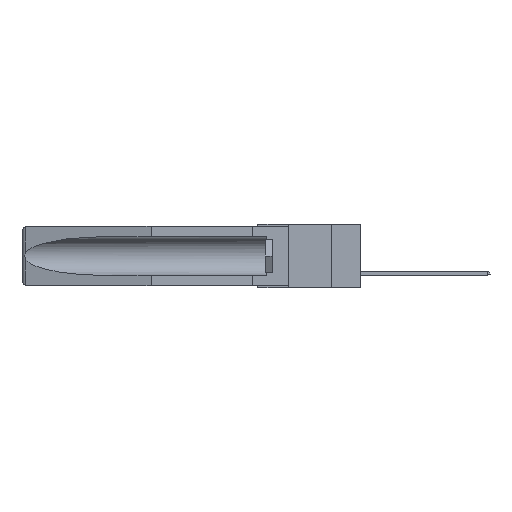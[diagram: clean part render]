
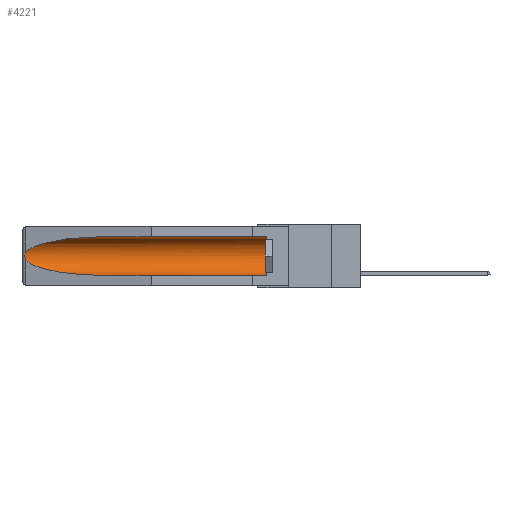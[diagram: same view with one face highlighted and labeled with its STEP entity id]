
A CAD part, left-side view. The second image highlights one B-rep face of the part: STEP entity #4221.
In plain terms, the highlighted cylindrical face has radius 2.857 mm (diameter 5.715 mm), a partial arc.
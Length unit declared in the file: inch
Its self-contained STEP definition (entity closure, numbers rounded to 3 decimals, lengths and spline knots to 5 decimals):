
#204 = VERTEX_POINT ( 'NONE', #32647 ) ;
#255 = EDGE_LOOP ( 'NONE', ( #9929, #26376, #19438, #7345, #10307, #28640 ) ) ;
#1029 = CARTESIAN_POINT ( 'NONE',  ( 0.26655, 1.53094, -0.18657 ) ) ;
#1532 =( BOUNDED_CURVE ( )  B_SPLINE_CURVE ( 3, ( #26139, #7770, #10874, #23546 ),
 .UNSPECIFIED., .F., .F. ) 
 B_SPLINE_CURVE_WITH_KNOTS ( ( 4, 4 ),
 ( 4.71239, 6.08839 ),
 .UNSPECIFIED. ) 
 CURVE ( )  GEOMETRIC_REPRESENTATION_ITEM ( )  RATIONAL_B_SPLINE_CURVE ( ( 1., 0.848, 0.848, 1. ) ) 
 REPRESENTATION_ITEM ( '' )  );
#1711 = DIRECTION ( 'NONE',  ( 0., 0., 1. ) ) ;
#2578 =( BOUNDED_CURVE ( )  B_SPLINE_CURVE ( 3, ( #14577, #17457, #25139, #32264 ),
 .UNSPECIFIED., .F., .F. ) 
 B_SPLINE_CURVE_WITH_KNOTS ( ( 4, 4 ),
 ( 0.1948, 1.5708 ),
 .UNSPECIFIED. ) 
 CURVE ( )  GEOMETRIC_REPRESENTATION_ITEM ( )  RATIONAL_B_SPLINE_CURVE ( ( 1., 0.848, 0.848, 1. ) ) 
 REPRESENTATION_ITEM ( '' )  );
#3154 = VERTEX_POINT ( 'NONE', #9610 ) ;
#3548 = DIRECTION ( 'NONE',  ( 0., -1., 0. ) ) ;
#4221 = ADVANCED_FACE ( 'NONE', ( #26932 ), #6598, .F. ) ;
#6135 = DIRECTION ( 'NONE',  ( 0., 1., 0. ) ) ;
#6598 = CYLINDRICAL_SURFACE ( 'NONE', #27250, 0.1125 ) ;
#7075 = CARTESIAN_POINT ( 'NONE',  ( 0.155, 1.07973, -0.284 ) ) ;
#7345 = ORIENTED_EDGE ( 'NONE', *, *, #27409, .F. ) ;
#7770 = CARTESIAN_POINT ( 'NONE',  ( 0.21114, 1.30732, -0.059 ) ) ;
#8404 = VERTEX_POINT ( 'NONE', #16386 ) ;
#8827 = CARTESIAN_POINT ( 'NONE',  ( 0.26597, 1.52961, -0.15275 ) ) ;
#9610 = CARTESIAN_POINT ( 'NONE',  ( 0.155, 0.126, -0.284 ) ) ;
#9929 = ORIENTED_EDGE ( 'NONE', *, *, #29488, .T. ) ;
#10307 = ORIENTED_EDGE ( 'NONE', *, *, #11218, .T. ) ;
#10533 = CARTESIAN_POINT ( 'NONE',  ( 0.26537, 1.52718, -0.19328 ) ) ;
#10874 = CARTESIAN_POINT ( 'NONE',  ( 0.25451, 1.48313, -0.09465 ) ) ;
#11218 = EDGE_CURVE ( 'NONE', #3154, #31500, #13970, .T. ) ;
#11290 = CARTESIAN_POINT ( 'NONE',  ( 0.2675, 1.53308, -0.16763 ) ) ;
#12491 = VERTEX_POINT ( 'NONE', #10533 ) ;
#13742 = CARTESIAN_POINT ( 'NONE',  ( 0.26537, 1.52718, -0.14972 ) ) ;
#13970 = CIRCLE ( 'NONE', #29177, 0.1125 ) ;
#14577 = CARTESIAN_POINT ( 'NONE',  ( 0.26537, 1.52718, -0.19328 ) ) ;
#14756 = CARTESIAN_POINT ( 'NONE',  ( 0.155, -0.30754, -0.1715 ) ) ;
#16190 = CARTESIAN_POINT ( 'NONE',  ( 0.2673, 1.5327, -0.16383 ) ) ;
#16386 = CARTESIAN_POINT ( 'NONE',  ( 0.26537, 1.52718, -0.14972 ) ) ;
#16401 = CARTESIAN_POINT ( 'NONE',  ( 0.26537, 1.52718, -0.19328 ) ) ;
#16489 = CARTESIAN_POINT ( 'NONE',  ( 0.155, -0.30754, -0.059 ) ) ;
#17457 = CARTESIAN_POINT ( 'NONE',  ( 0.25451, 1.48313, -0.24835 ) ) ;
#18757 = CARTESIAN_POINT ( 'NONE',  ( 0.26597, 1.5296, -0.19026 ) ) ;
#19438 = ORIENTED_EDGE ( 'NONE', *, *, #19830, .T. ) ;
#19830 = EDGE_CURVE ( 'NONE', #12491, #29817, #2578, .T. ) ;
#20672 = EDGE_CURVE ( 'NONE', #8404, #12491, #29696, .T. ) ;
#21003 = LINE ( 'NONE', #29804, #30559 ) ;
#21214 = EDGE_CURVE ( 'NONE', #31500, #204, #29414, .T. ) ;
#22615 = CARTESIAN_POINT ( 'NONE',  ( 0.155, 0.126, -0.059 ) ) ;
#23546 = CARTESIAN_POINT ( 'NONE',  ( 0.26537, 1.52718, -0.14972 ) ) ;
#25139 = CARTESIAN_POINT ( 'NONE',  ( 0.21114, 1.30732, -0.284 ) ) ;
#26139 = CARTESIAN_POINT ( 'NONE',  ( 0.155, 1.07973, -0.059 ) ) ;
#26269 = CARTESIAN_POINT ( 'NONE',  ( 0.155, 0.126, -0.1715 ) ) ;
#26330 = CARTESIAN_POINT ( 'NONE',  ( 0.26654, 1.53092, -0.15636 ) ) ;
#26376 = ORIENTED_EDGE ( 'NONE', *, *, #20672, .T. ) ;
#26669 = CARTESIAN_POINT ( 'NONE',  ( 0.2675, 1.53308, -0.17534 ) ) ;
#26932 = FACE_OUTER_BOUND ( 'NONE', #255, .T. ) ;
#27250 = AXIS2_PLACEMENT_3D ( 'NONE', #14756, #32218, #1711 ) ;
#27409 = EDGE_CURVE ( 'NONE', #3154, #29817, #21003, .T. ) ;
#28640 = ORIENTED_EDGE ( 'NONE', *, *, #21214, .T. ) ;
#28822 = DIRECTION ( 'NONE',  ( 0., 0., 1. ) ) ;
#29177 = AXIS2_PLACEMENT_3D ( 'NONE', #26269, #3548, #28822 ) ;
#29414 = LINE ( 'NONE', #16489, #31031 ) ;
#29488 = EDGE_CURVE ( 'NONE', #204, #8404, #1532, .T. ) ;
#29572 = DIRECTION ( 'NONE',  ( 0., 1., 0. ) ) ;
#29696 = B_SPLINE_CURVE_WITH_KNOTS ( 'NONE', 3,
 ( #13742, #8827, #26330, #16190, #11290, #26669, #31547, #1029, #18757, #16401 ),
 .UNSPECIFIED., .F., .F.,
 ( 4, 2, 2, 2, 4 ),
 ( 0., 0.00029, 0.00058, 0.00087, 0.00117 ),
 .UNSPECIFIED. ) ;
#29804 = CARTESIAN_POINT ( 'NONE',  ( 0.155, -0.30754, -0.284 ) ) ;
#29817 = VERTEX_POINT ( 'NONE', #7075 ) ;
#30559 = VECTOR ( 'NONE', #29572, 39.37008 ) ;
#31031 = VECTOR ( 'NONE', #6135, 39.37008 ) ;
#31500 = VERTEX_POINT ( 'NONE', #22615 ) ;
#31547 = CARTESIAN_POINT ( 'NONE',  ( 0.2673, 1.53269, -0.17917 ) ) ;
#32218 = DIRECTION ( 'NONE',  ( 0., 1., 0. ) ) ;
#32264 = CARTESIAN_POINT ( 'NONE',  ( 0.155, 1.07973, -0.284 ) ) ;
#32647 = CARTESIAN_POINT ( 'NONE',  ( 0.155, 1.07973, -0.059 ) ) ;
